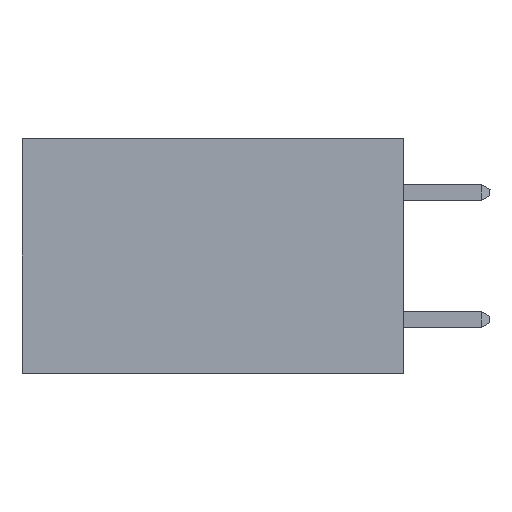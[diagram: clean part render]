
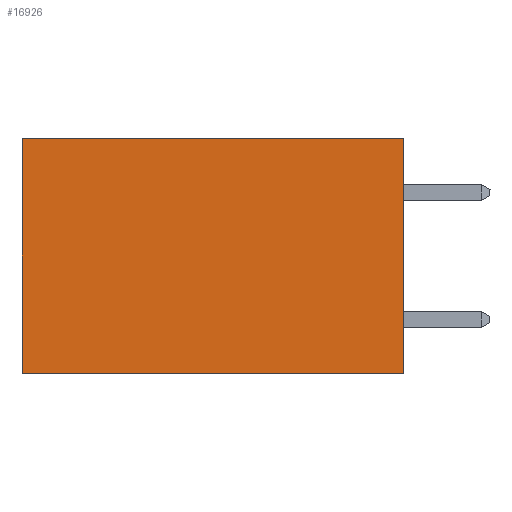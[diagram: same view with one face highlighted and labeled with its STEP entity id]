
A CAD part, left-side view. The second image highlights one B-rep face of the part: STEP entity #16926.
In plain terms, the highlighted planar face has unit normal (-1, 0, 0).
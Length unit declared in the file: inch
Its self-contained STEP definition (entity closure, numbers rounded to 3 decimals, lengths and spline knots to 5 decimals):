
#413 = PLANE ( 'NONE',  #10583 ) ;
#555 = ORIENTED_EDGE ( 'NONE', *, *, #6333, .T. ) ;
#1323 = EDGE_CURVE ( 'NONE', #15205, #3746, #10022, .T. ) ;
#1971 = DIRECTION ( 'NONE',  ( 0., 0., -1. ) ) ;
#2332 = LINE ( 'NONE', #13006, #13569 ) ;
#3746 = VERTEX_POINT ( 'NONE', #13960 ) ;
#3883 = VECTOR ( 'NONE', #13437, 39.37008 ) ;
#5038 = VERTEX_POINT ( 'NONE', #5499 ) ;
#5499 = CARTESIAN_POINT ( 'NONE',  ( 0.2875, 0.6, 0. ) ) ;
#5773 = DIRECTION ( 'NONE',  ( 0., 1., 0. ) ) ;
#6333 = EDGE_CURVE ( 'NONE', #5038, #7381, #10551, .T. ) ;
#6925 = EDGE_CURVE ( 'NONE', #15205, #5038, #7815, .T. ) ;
#7381 = VERTEX_POINT ( 'NONE', #13016 ) ;
#7485 = DIRECTION ( 'NONE',  ( 0., 0., -1. ) ) ;
#7815 = LINE ( 'NONE', #16885, #3883 ) ;
#9676 = FACE_OUTER_BOUND ( 'NONE', #10416, .T. ) ;
#9969 = CARTESIAN_POINT ( 'NONE',  ( 0.2875, 0., 0. ) ) ;
#10022 = LINE ( 'NONE', #9969, #17284 ) ;
#10416 = EDGE_LOOP ( 'NONE', ( #555, #16777, #16330, #10956 ) ) ;
#10551 = LINE ( 'NONE', #11541, #13944 ) ;
#10583 = AXIS2_PLACEMENT_3D ( 'NONE', #12195, #10797, #1971 ) ;
#10797 = DIRECTION ( 'NONE',  ( 1., 0., 0. ) ) ;
#10956 = ORIENTED_EDGE ( 'NONE', *, *, #6925, .T. ) ;
#11541 = CARTESIAN_POINT ( 'NONE',  ( 0.2875, 0.6, 0. ) ) ;
#12195 = CARTESIAN_POINT ( 'NONE',  ( 0.2875, 0., 0. ) ) ;
#13006 = CARTESIAN_POINT ( 'NONE',  ( 0.2875, 0., -0.37 ) ) ;
#13016 = CARTESIAN_POINT ( 'NONE',  ( 0.2875, 0.6, -0.37 ) ) ;
#13437 = DIRECTION ( 'NONE',  ( 0., 1., 0. ) ) ;
#13569 = VECTOR ( 'NONE', #5773, 39.37008 ) ;
#13944 = VECTOR ( 'NONE', #7485, 39.37008 ) ;
#13960 = CARTESIAN_POINT ( 'NONE',  ( 0.2875, 0., -0.37 ) ) ;
#15205 = VERTEX_POINT ( 'NONE', #15817 ) ;
#15555 = DIRECTION ( 'NONE',  ( 0., 0., -1. ) ) ;
#15745 = EDGE_CURVE ( 'NONE', #3746, #7381, #2332, .T. ) ;
#15817 = CARTESIAN_POINT ( 'NONE',  ( 0.2875, 0., 0. ) ) ;
#16330 = ORIENTED_EDGE ( 'NONE', *, *, #1323, .F. ) ;
#16777 = ORIENTED_EDGE ( 'NONE', *, *, #15745, .F. ) ;
#16885 = CARTESIAN_POINT ( 'NONE',  ( 0.2875, 0., 0. ) ) ;
#16926 = ADVANCED_FACE ( 'NONE', ( #9676 ), #413, .F. ) ;
#17284 = VECTOR ( 'NONE', #15555, 39.37008 ) ;
